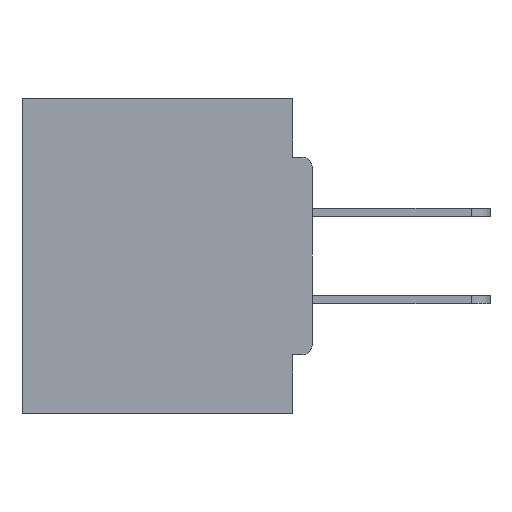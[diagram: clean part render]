
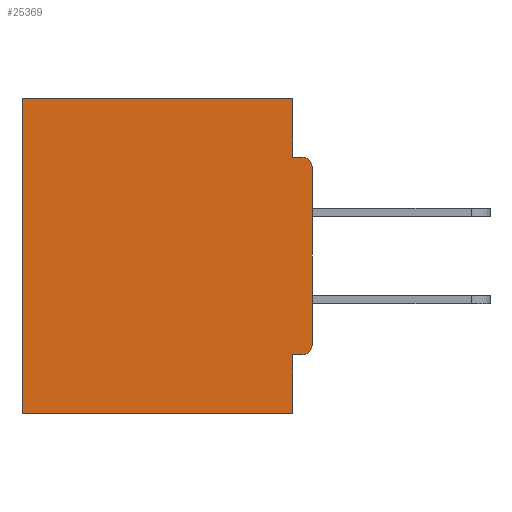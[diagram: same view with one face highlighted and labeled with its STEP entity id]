
A CAD part, left-side view. The second image highlights one B-rep face of the part: STEP entity #25369.
In plain terms, the highlighted planar face has unit normal (-1, 0, 0).
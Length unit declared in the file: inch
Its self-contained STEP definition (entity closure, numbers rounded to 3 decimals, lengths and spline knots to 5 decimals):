
#205 = CARTESIAN_POINT ( 'NONE',  ( 0.298, 0.46, 0. ) ) ;
#317 = VERTEX_POINT ( 'NONE', #30409 ) ;
#599 = LINE ( 'NONE', #2538, #19214 ) ;
#1346 = EDGE_CURVE ( 'NONE', #24603, #317, #3319, .T. ) ;
#2086 = DIRECTION ( 'NONE',  ( 0., 0., -1. ) ) ;
#2198 = EDGE_CURVE ( 'NONE', #27784, #32897, #32137, .T. ) ;
#2538 = CARTESIAN_POINT ( 'NONE',  ( 0.298, 0., 0. ) ) ;
#2929 = FACE_OUTER_BOUND ( 'NONE', #15856, .T. ) ;
#3030 = VECTOR ( 'NONE', #21343, 39.37008 ) ;
#3319 = LINE ( 'NONE', #25090, #28948 ) ;
#3692 = CARTESIAN_POINT ( 'NONE',  ( 0.298, 0.031, -0.0935 ) ) ;
#3940 = AXIS2_PLACEMENT_3D ( 'NONE', #23451, #7872, #12627 ) ;
#4041 = AXIS2_PLACEMENT_3D ( 'NONE', #24042, #31668, #13654 ) ;
#5489 = CARTESIAN_POINT ( 'NONE',  ( 0.298, 0.015, -0.3915 ) ) ;
#5693 = CARTESIAN_POINT ( 'NONE',  ( 0.298, 0., 0. ) ) ;
#6255 = LINE ( 'NONE', #16648, #3030 ) ;
#6637 = VECTOR ( 'NONE', #26157, 39.37008 ) ;
#7442 = CARTESIAN_POINT ( 'NONE',  ( 0.298, 0.015, -0.0935 ) ) ;
#7666 = DIRECTION ( 'NONE',  ( 0., -1., 0. ) ) ;
#7872 = DIRECTION ( 'NONE',  ( 1., 0., 0. ) ) ;
#8408 = DIRECTION ( 'NONE',  ( 0., 0., -1. ) ) ;
#8466 = ORIENTED_EDGE ( 'NONE', *, *, #1346, .F. ) ;
#9720 = CARTESIAN_POINT ( 'NONE',  ( 0.298, 0., -0.3915 ) ) ;
#10037 = AXIS2_PLACEMENT_3D ( 'NONE', #5489, #11151, #26312 ) ;
#10155 = CARTESIAN_POINT ( 'NONE',  ( 0.298, 0., -0.0935 ) ) ;
#10355 = VERTEX_POINT ( 'NONE', #29386 ) ;
#10425 = CARTESIAN_POINT ( 'NONE',  ( 0.298, 0.031, -0.5 ) ) ;
#10828 = CARTESIAN_POINT ( 'NONE',  ( 0.298, 0.015, -0.4065 ) ) ;
#10974 = DIRECTION ( 'NONE',  ( 0., 1., 0. ) ) ;
#11151 = DIRECTION ( 'NONE',  ( -1., 0., 0. ) ) ;
#12018 = CIRCLE ( 'NONE', #10037, 0.015 ) ;
#12257 = VERTEX_POINT ( 'NONE', #9720 ) ;
#12627 = DIRECTION ( 'NONE',  ( 0., 0., -1. ) ) ;
#13411 = EDGE_CURVE ( 'NONE', #24603, #12257, #12018, .T. ) ;
#13654 = DIRECTION ( 'NONE',  ( 0., 0., -1. ) ) ;
#14110 = ORIENTED_EDGE ( 'NONE', *, *, #30410, .F. ) ;
#15027 = EDGE_CURVE ( 'NONE', #29062, #19890, #26620, .T. ) ;
#15094 = EDGE_CURVE ( 'NONE', #19890, #32897, #6255, .T. ) ;
#15124 = PLANE ( 'NONE',  #3940 ) ;
#15856 = EDGE_LOOP ( 'NONE', ( #22401, #24415, #16774, #23491, #28124, #28479, #14110, #8466, #20330, #26562 ) ) ;
#15966 = VECTOR ( 'NONE', #7666, 39.37008 ) ;
#16104 = CARTESIAN_POINT ( 'NONE',  ( 0.298, 0.031, -0.5 ) ) ;
#16648 = CARTESIAN_POINT ( 'NONE',  ( 0.298, 0.46, 0. ) ) ;
#16695 = EDGE_CURVE ( 'NONE', #10355, #21873, #26075, .T. ) ;
#16774 = ORIENTED_EDGE ( 'NONE', *, *, #32583, .F. ) ;
#18006 = CARTESIAN_POINT ( 'NONE',  ( 0.298, 0.46, -0.5 ) ) ;
#18945 = LINE ( 'NONE', #16104, #23430 ) ;
#19214 = VECTOR ( 'NONE', #28868, 39.37008 ) ;
#19890 = VERTEX_POINT ( 'NONE', #205 ) ;
#20330 = ORIENTED_EDGE ( 'NONE', *, *, #13411, .T. ) ;
#21343 = DIRECTION ( 'NONE',  ( 0., 0., -1. ) ) ;
#21873 = VERTEX_POINT ( 'NONE', #7442 ) ;
#22401 = ORIENTED_EDGE ( 'NONE', *, *, #16695, .T. ) ;
#22632 = VERTEX_POINT ( 'NONE', #3692 ) ;
#23283 = CARTESIAN_POINT ( 'NONE',  ( 0.298, 0.031, 0. ) ) ;
#23430 = VECTOR ( 'NONE', #8408, 39.37008 ) ;
#23451 = CARTESIAN_POINT ( 'NONE',  ( 0.298, 0., 0. ) ) ;
#23491 = ORIENTED_EDGE ( 'NONE', *, *, #15027, .T. ) ;
#24042 = CARTESIAN_POINT ( 'NONE',  ( 0.298, 0.015, -0.1085 ) ) ;
#24415 = ORIENTED_EDGE ( 'NONE', *, *, #29786, .F. ) ;
#24603 = VERTEX_POINT ( 'NONE', #10828 ) ;
#24766 = DIRECTION ( 'NONE',  ( 0., 1., 0. ) ) ;
#24893 = CARTESIAN_POINT ( 'NONE',  ( 0.298, 0., -0.5 ) ) ;
#25090 = CARTESIAN_POINT ( 'NONE',  ( 0.298, 0., -0.4065 ) ) ;
#25345 = CARTESIAN_POINT ( 'NONE',  ( 0.298, 0.031, -0.5 ) ) ;
#25369 = ADVANCED_FACE ( 'NONE', ( #2929 ), #15124, .F. ) ;
#26075 = CIRCLE ( 'NONE', #4041, 0.015 ) ;
#26157 = DIRECTION ( 'NONE',  ( 0., 1., 0. ) ) ;
#26312 = DIRECTION ( 'NONE',  ( 0., 0., -1. ) ) ;
#26562 = ORIENTED_EDGE ( 'NONE', *, *, #30526, .F. ) ;
#26620 = LINE ( 'NONE', #5693, #6637 ) ;
#26621 = VECTOR ( 'NONE', #2086, 39.37008 ) ;
#26859 = VECTOR ( 'NONE', #24766, 39.37008 ) ;
#27387 = LINE ( 'NONE', #25345, #26621 ) ;
#27784 = VERTEX_POINT ( 'NONE', #10425 ) ;
#28124 = ORIENTED_EDGE ( 'NONE', *, *, #15094, .T. ) ;
#28479 = ORIENTED_EDGE ( 'NONE', *, *, #2198, .F. ) ;
#28868 = DIRECTION ( 'NONE',  ( 0., 0., -1. ) ) ;
#28948 = VECTOR ( 'NONE', #10974, 39.37008 ) ;
#29062 = VERTEX_POINT ( 'NONE', #23283 ) ;
#29386 = CARTESIAN_POINT ( 'NONE',  ( 0.298, 0., -0.1085 ) ) ;
#29786 = EDGE_CURVE ( 'NONE', #22632, #21873, #29843, .T. ) ;
#29843 = LINE ( 'NONE', #10155, #15966 ) ;
#30409 = CARTESIAN_POINT ( 'NONE',  ( 0.298, 0.031, -0.4065 ) ) ;
#30410 = EDGE_CURVE ( 'NONE', #317, #27784, #27387, .T. ) ;
#30526 = EDGE_CURVE ( 'NONE', #10355, #12257, #599, .T. ) ;
#31668 = DIRECTION ( 'NONE',  ( -1., 0., 0. ) ) ;
#32137 = LINE ( 'NONE', #24893, #26859 ) ;
#32583 = EDGE_CURVE ( 'NONE', #29062, #22632, #18945, .T. ) ;
#32897 = VERTEX_POINT ( 'NONE', #18006 ) ;
